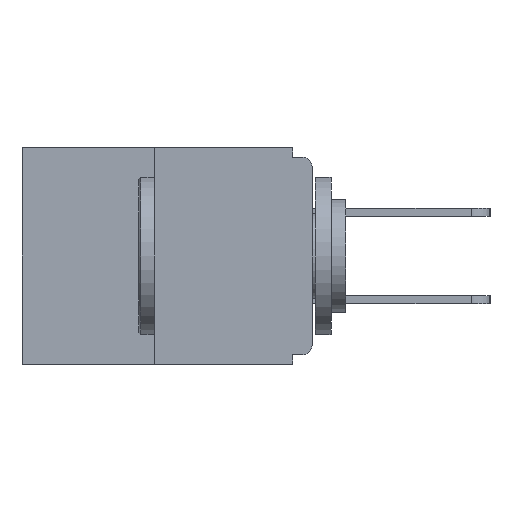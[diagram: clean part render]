
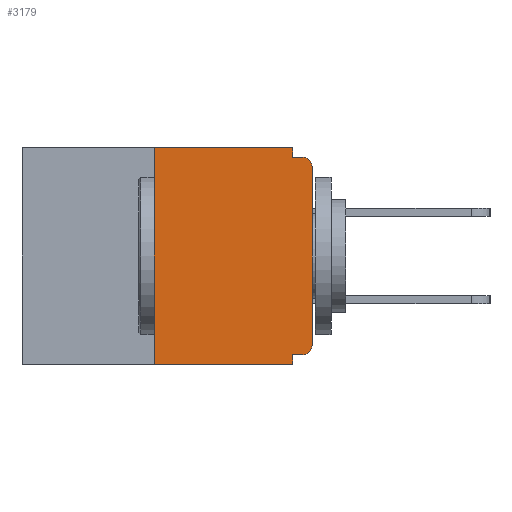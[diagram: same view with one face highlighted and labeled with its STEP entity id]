
A CAD part, left-side view. The second image highlights one B-rep face of the part: STEP entity #3179.
In plain terms, the highlighted planar face has unit normal (-1, 0, 0).
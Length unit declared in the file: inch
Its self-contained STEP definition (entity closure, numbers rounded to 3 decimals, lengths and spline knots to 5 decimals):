
#71 = VERTEX_POINT ( 'NONE', #9128 ) ;
#523 = DIRECTION ( 'NONE',  ( 0., 1., 0. ) ) ;
#874 = CARTESIAN_POINT ( 'NONE',  ( 0., 0.46, 0. ) ) ;
#913 = DIRECTION ( 'NONE',  ( 0., 0., -1. ) ) ;
#952 = VERTEX_POINT ( 'NONE', #10881 ) ;
#1064 = EDGE_CURVE ( 'NONE', #952, #12655, #11890, .T. ) ;
#1197 = AXIS2_PLACEMENT_3D ( 'NONE', #1471, #11728, #12130 ) ;
#1245 = CARTESIAN_POINT ( 'NONE',  ( 0., 0.031, -0.015 ) ) ;
#1289 = LINE ( 'NONE', #15417, #2235 ) ;
#1471 = CARTESIAN_POINT ( 'NONE',  ( 0., 0.015, -0.313 ) ) ;
#1497 = VERTEX_POINT ( 'NONE', #3072 ) ;
#2050 = CARTESIAN_POINT ( 'NONE',  ( 0., 0.25, 0. ) ) ;
#2153 = DIRECTION ( 'NONE',  ( 0., 0., 1. ) ) ;
#2235 = VECTOR ( 'NONE', #16962, 39.37008 ) ;
#2238 = ORIENTED_EDGE ( 'NONE', *, *, #15919, .T. ) ;
#2582 = EDGE_LOOP ( 'NONE', ( #5058, #3424, #14029, #15133, #4628, #7851, #14327, #2238, #5494, #17786 ) ) ;
#2655 = CARTESIAN_POINT ( 'NONE',  ( 0., 0.015, -0.015 ) ) ;
#2907 = VERTEX_POINT ( 'NONE', #2050 ) ;
#3072 = CARTESIAN_POINT ( 'NONE',  ( 0., 0., -0.313 ) ) ;
#3179 = ADVANCED_FACE ( 'NONE', ( #4236 ), #6989, .F. ) ;
#3424 = ORIENTED_EDGE ( 'NONE', *, *, #9896, .F. ) ;
#3603 = CARTESIAN_POINT ( 'NONE',  ( 0., 0.25, -0.343 ) ) ;
#4236 = FACE_OUTER_BOUND ( 'NONE', #2582, .T. ) ;
#4290 = CARTESIAN_POINT ( 'NONE',  ( 0., 0.031, -0.343 ) ) ;
#4317 = AXIS2_PLACEMENT_3D ( 'NONE', #11297, #17764, #913 ) ;
#4628 = ORIENTED_EDGE ( 'NONE', *, *, #1064, .F. ) ;
#5058 = ORIENTED_EDGE ( 'NONE', *, *, #7809, .F. ) ;
#5282 = VECTOR ( 'NONE', #12213, 39.37008 ) ;
#5494 = ORIENTED_EDGE ( 'NONE', *, *, #12198, .F. ) ;
#5621 = EDGE_CURVE ( 'NONE', #12655, #16103, #1289, .T. ) ;
#5736 = VECTOR ( 'NONE', #15054, 39.37008 ) ;
#6938 = EDGE_CURVE ( 'NONE', #16468, #16103, #19054, .T. ) ;
#6989 = PLANE ( 'NONE',  #10658 ) ;
#7024 = CARTESIAN_POINT ( 'NONE',  ( 0., 0.46, -0.343 ) ) ;
#7038 = VECTOR ( 'NONE', #9254, 39.37008 ) ;
#7809 = EDGE_CURVE ( 'NONE', #2907, #71, #11132, .T. ) ;
#7851 = ORIENTED_EDGE ( 'NONE', *, *, #19311, .T. ) ;
#7902 = VERTEX_POINT ( 'NONE', #2655 ) ;
#8292 = VECTOR ( 'NONE', #523, 39.37008 ) ;
#8492 = DIRECTION ( 'NONE',  ( 0., -1., 0. ) ) ;
#8936 = VECTOR ( 'NONE', #8492, 39.37008 ) ;
#9128 = CARTESIAN_POINT ( 'NONE',  ( 0., 0.031, 0. ) ) ;
#9254 = DIRECTION ( 'NONE',  ( 0., 0., -1. ) ) ;
#9295 = VERTEX_POINT ( 'NONE', #9343 ) ;
#9343 = CARTESIAN_POINT ( 'NONE',  ( 0., 0., -0.03 ) ) ;
#9404 = CARTESIAN_POINT ( 'NONE',  ( 0., 0., -0.328 ) ) ;
#9638 = CARTESIAN_POINT ( 'NONE',  ( 0., 0.031, -0.328 ) ) ;
#9896 = EDGE_CURVE ( 'NONE', #16468, #2907, #17393, .T. ) ;
#10018 = CIRCLE ( 'NONE', #1197, 0.015 ) ;
#10653 = EDGE_CURVE ( 'NONE', #1497, #9295, #14495, .T. ) ;
#10658 = AXIS2_PLACEMENT_3D ( 'NONE', #874, #17518, #11455 ) ;
#10730 = CARTESIAN_POINT ( 'NONE',  ( 0., 0.25, 0. ) ) ;
#10737 = CARTESIAN_POINT ( 'NONE',  ( 0., 0.031, 0. ) ) ;
#10881 = CARTESIAN_POINT ( 'NONE',  ( 0., 0.015, -0.328 ) ) ;
#11077 = LINE ( 'NONE', #10737, #7038 ) ;
#11132 = LINE ( 'NONE', #11381, #8936 ) ;
#11176 = DIRECTION ( 'NONE',  ( 0., -1., 0. ) ) ;
#11192 = VECTOR ( 'NONE', #2153, 39.37008 ) ;
#11297 = CARTESIAN_POINT ( 'NONE',  ( 0., 0.015, -0.03 ) ) ;
#11381 = CARTESIAN_POINT ( 'NONE',  ( 0., 0.46, 0. ) ) ;
#11455 = DIRECTION ( 'NONE',  ( 0., 0., -1. ) ) ;
#11728 = DIRECTION ( 'NONE',  ( -1., 0., 0. ) ) ;
#11890 = LINE ( 'NONE', #9404, #8292 ) ;
#12130 = DIRECTION ( 'NONE',  ( 0., 0., -1. ) ) ;
#12198 = EDGE_CURVE ( 'NONE', #18960, #7902, #14664, .T. ) ;
#12213 = DIRECTION ( 'NONE',  ( 0., 0., 1. ) ) ;
#12655 = VERTEX_POINT ( 'NONE', #9638 ) ;
#12681 = CARTESIAN_POINT ( 'NONE',  ( 0., 0., 0. ) ) ;
#14029 = ORIENTED_EDGE ( 'NONE', *, *, #6938, .T. ) ;
#14224 = CARTESIAN_POINT ( 'NONE',  ( 0., 0., -0.015 ) ) ;
#14327 = ORIENTED_EDGE ( 'NONE', *, *, #10653, .T. ) ;
#14495 = LINE ( 'NONE', #12681, #11192 ) ;
#14664 = LINE ( 'NONE', #14224, #15890 ) ;
#15054 = DIRECTION ( 'NONE',  ( 0., -1., 0. ) ) ;
#15133 = ORIENTED_EDGE ( 'NONE', *, *, #5621, .F. ) ;
#15417 = CARTESIAN_POINT ( 'NONE',  ( 0., 0.031, -0.343 ) ) ;
#15890 = VECTOR ( 'NONE', #11176, 39.37008 ) ;
#15919 = EDGE_CURVE ( 'NONE', #9295, #7902, #16125, .T. ) ;
#16103 = VERTEX_POINT ( 'NONE', #4290 ) ;
#16125 = CIRCLE ( 'NONE', #4317, 0.015 ) ;
#16296 = EDGE_CURVE ( 'NONE', #71, #18960, #11077, .T. ) ;
#16468 = VERTEX_POINT ( 'NONE', #3603 ) ;
#16962 = DIRECTION ( 'NONE',  ( 0., 0., -1. ) ) ;
#17393 = LINE ( 'NONE', #10730, #5282 ) ;
#17518 = DIRECTION ( 'NONE',  ( 1., 0., 0. ) ) ;
#17764 = DIRECTION ( 'NONE',  ( -1., 0., 0. ) ) ;
#17786 = ORIENTED_EDGE ( 'NONE', *, *, #16296, .F. ) ;
#18960 = VERTEX_POINT ( 'NONE', #1245 ) ;
#19054 = LINE ( 'NONE', #7024, #5736 ) ;
#19311 = EDGE_CURVE ( 'NONE', #952, #1497, #10018, .T. ) ;
